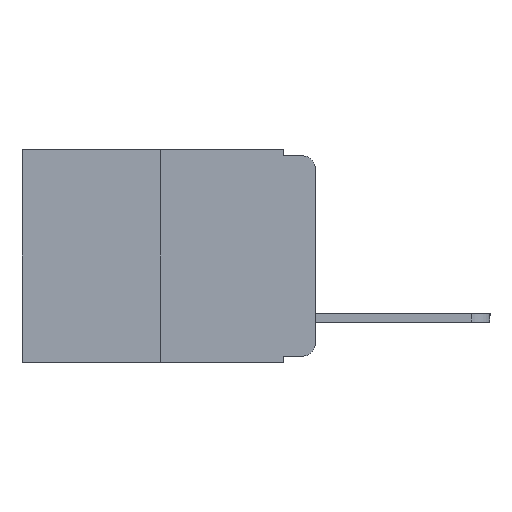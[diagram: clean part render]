
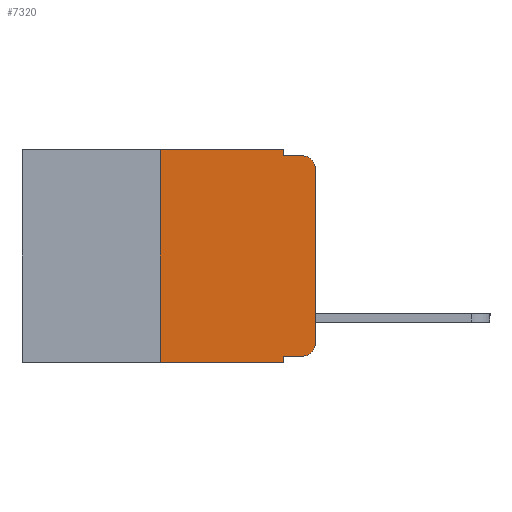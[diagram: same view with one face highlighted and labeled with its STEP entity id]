
A CAD part, left-side view. The second image highlights one B-rep face of the part: STEP entity #7320.
In plain terms, the highlighted planar face has unit normal (-1, 0, 0).
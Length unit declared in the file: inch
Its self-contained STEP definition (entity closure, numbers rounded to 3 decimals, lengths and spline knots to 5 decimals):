
#650 = VECTOR ( 'NONE', #7055, 39.37008 ) ;
#966 = CARTESIAN_POINT ( 'NONE',  ( 0., 0.473, 0. ) ) ;
#993 = DIRECTION ( 'NONE',  ( 0., -1., 0. ) ) ;
#1470 = DIRECTION ( 'NONE',  ( -1., 0., 0. ) ) ;
#1630 = VECTOR ( 'NONE', #1976, 39.37008 ) ;
#1656 = CARTESIAN_POINT ( 'NONE',  ( 0., 0.051, -0.333 ) ) ;
#1976 = DIRECTION ( 'NONE',  ( 0., 0., 1. ) ) ;
#2363 = LINE ( 'NONE', #966, #13123 ) ;
#2447 = AXIS2_PLACEMENT_3D ( 'NONE', #13130, #1470, #10082 ) ;
#2453 = VECTOR ( 'NONE', #11884, 39.37008 ) ;
#2744 = DIRECTION ( 'NONE',  ( 0., 0., -1. ) ) ;
#3131 = DIRECTION ( 'NONE',  ( 0., -1., 0. ) ) ;
#3167 = PLANE ( 'NONE',  #14498 ) ;
#3228 = DIRECTION ( 'NONE',  ( -1., 0., 0. ) ) ;
#3326 = VERTEX_POINT ( 'NONE', #13422 ) ;
#3493 = EDGE_CURVE ( 'NONE', #12688, #3326, #14254, .T. ) ;
#4221 = VERTEX_POINT ( 'NONE', #12447 ) ;
#4460 = VERTEX_POINT ( 'NONE', #9990 ) ;
#4807 = CIRCLE ( 'NONE', #2447, 0.02 ) ;
#5131 = EDGE_CURVE ( 'NONE', #18100, #12276, #2363, .T. ) ;
#5976 = CARTESIAN_POINT ( 'NONE',  ( 0., 0.25, 0. ) ) ;
#6099 = EDGE_CURVE ( 'NONE', #11650, #18100, #16963, .T. ) ;
#6119 = VECTOR ( 'NONE', #2744, 39.37008 ) ;
#6581 = LINE ( 'NONE', #16670, #6119 ) ;
#7011 = CARTESIAN_POINT ( 'NONE',  ( 0., 0.473, -0.343 ) ) ;
#7055 = DIRECTION ( 'NONE',  ( 0., 0., 1. ) ) ;
#7320 = ADVANCED_FACE ( 'NONE', ( #8894 ), #3167, .F. ) ;
#7427 = CARTESIAN_POINT ( 'NONE',  ( 0., 0.051, -0.01 ) ) ;
#7461 = DIRECTION ( 'NONE',  ( 1., 0., 0. ) ) ;
#7488 = ORIENTED_EDGE ( 'NONE', *, *, #5131, .F. ) ;
#7681 = LINE ( 'NONE', #7427, #14851 ) ;
#7697 = ORIENTED_EDGE ( 'NONE', *, *, #7761, .T. ) ;
#7714 = EDGE_LOOP ( 'NONE', ( #7697, #12090, #13799, #17828, #7488, #8790, #12851, #10126, #13700, #14141 ) ) ;
#7761 = EDGE_CURVE ( 'NONE', #15585, #12688, #11987, .T. ) ;
#8402 = DIRECTION ( 'NONE',  ( 0., -1., 0. ) ) ;
#8790 = ORIENTED_EDGE ( 'NONE', *, *, #6099, .F. ) ;
#8894 = FACE_OUTER_BOUND ( 'NONE', #7714, .T. ) ;
#9093 = EDGE_CURVE ( 'NONE', #4221, #15585, #4807, .T. ) ;
#9990 = CARTESIAN_POINT ( 'NONE',  ( 0., 0.051, -0.01 ) ) ;
#10082 = DIRECTION ( 'NONE',  ( 0., 0., -1. ) ) ;
#10126 = ORIENTED_EDGE ( 'NONE', *, *, #11890, .F. ) ;
#10583 = EDGE_CURVE ( 'NONE', #12276, #4460, #17656, .T. ) ;
#10609 = CARTESIAN_POINT ( 'NONE',  ( 0., 0.051, -0.343 ) ) ;
#11392 = VECTOR ( 'NONE', #8402, 39.37008 ) ;
#11472 = CARTESIAN_POINT ( 'NONE',  ( 0., 0., -0.313 ) ) ;
#11475 = DIRECTION ( 'NONE',  ( 0., -1., 0. ) ) ;
#11595 = VERTEX_POINT ( 'NONE', #13582 ) ;
#11628 = DIRECTION ( 'NONE',  ( 0., 0., -1. ) ) ;
#11650 = VERTEX_POINT ( 'NONE', #12118 ) ;
#11675 = CARTESIAN_POINT ( 'NONE',  ( 0., 0., -0.03 ) ) ;
#11884 = DIRECTION ( 'NONE',  ( 0., 0., -1. ) ) ;
#11890 = EDGE_CURVE ( 'NONE', #11595, #14834, #6581, .T. ) ;
#11987 = LINE ( 'NONE', #16400, #650 ) ;
#12090 = ORIENTED_EDGE ( 'NONE', *, *, #3493, .T. ) ;
#12118 = CARTESIAN_POINT ( 'NONE',  ( 0., 0.25, -0.343 ) ) ;
#12276 = VERTEX_POINT ( 'NONE', #16120 ) ;
#12296 = VECTOR ( 'NONE', #3131, 39.37008 ) ;
#12447 = CARTESIAN_POINT ( 'NONE',  ( 0., 0.02, -0.333 ) ) ;
#12688 = VERTEX_POINT ( 'NONE', #11675 ) ;
#12810 = DIRECTION ( 'NONE',  ( 0., 0., -1. ) ) ;
#12851 = ORIENTED_EDGE ( 'NONE', *, *, #16481, .T. ) ;
#12986 = CARTESIAN_POINT ( 'NONE',  ( 0., 0.02, -0.03 ) ) ;
#13123 = VECTOR ( 'NONE', #993, 39.37008 ) ;
#13130 = CARTESIAN_POINT ( 'NONE',  ( 0., 0.02, -0.313 ) ) ;
#13422 = CARTESIAN_POINT ( 'NONE',  ( 0., 0.02, -0.01 ) ) ;
#13425 = AXIS2_PLACEMENT_3D ( 'NONE', #12986, #3228, #11628 ) ;
#13582 = CARTESIAN_POINT ( 'NONE',  ( 0., 0.051, -0.333 ) ) ;
#13700 = ORIENTED_EDGE ( 'NONE', *, *, #15594, .T. ) ;
#13799 = ORIENTED_EDGE ( 'NONE', *, *, #15189, .F. ) ;
#14141 = ORIENTED_EDGE ( 'NONE', *, *, #9093, .T. ) ;
#14254 = CIRCLE ( 'NONE', #13425, 0.02 ) ;
#14498 = AXIS2_PLACEMENT_3D ( 'NONE', #17475, #7461, #12810 ) ;
#14512 = CARTESIAN_POINT ( 'NONE',  ( 0., 0.25, 0. ) ) ;
#14626 = CARTESIAN_POINT ( 'NONE',  ( 0., 0.051, 0. ) ) ;
#14834 = VERTEX_POINT ( 'NONE', #10609 ) ;
#14851 = VECTOR ( 'NONE', #11475, 39.37008 ) ;
#15189 = EDGE_CURVE ( 'NONE', #4460, #3326, #7681, .T. ) ;
#15455 = LINE ( 'NONE', #7011, #11392 ) ;
#15585 = VERTEX_POINT ( 'NONE', #11472 ) ;
#15594 = EDGE_CURVE ( 'NONE', #11595, #4221, #16375, .T. ) ;
#16120 = CARTESIAN_POINT ( 'NONE',  ( 0., 0.051, 0. ) ) ;
#16375 = LINE ( 'NONE', #1656, #12296 ) ;
#16400 = CARTESIAN_POINT ( 'NONE',  ( 0., 0., 0. ) ) ;
#16481 = EDGE_CURVE ( 'NONE', #11650, #14834, #15455, .T. ) ;
#16670 = CARTESIAN_POINT ( 'NONE',  ( 0., 0.051, 0. ) ) ;
#16963 = LINE ( 'NONE', #5976, #1630 ) ;
#17475 = CARTESIAN_POINT ( 'NONE',  ( 0., 0.473, 0. ) ) ;
#17656 = LINE ( 'NONE', #14626, #2453 ) ;
#17828 = ORIENTED_EDGE ( 'NONE', *, *, #10583, .F. ) ;
#18100 = VERTEX_POINT ( 'NONE', #14512 ) ;
